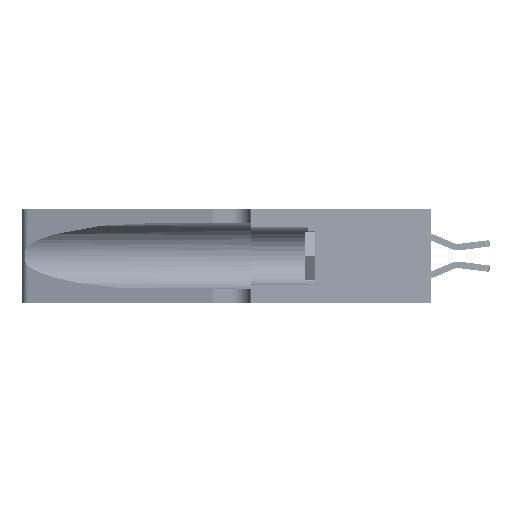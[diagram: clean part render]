
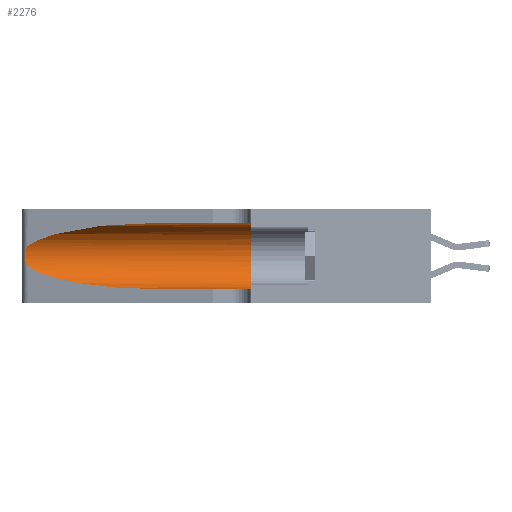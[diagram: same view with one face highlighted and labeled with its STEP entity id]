
A CAD part, left-side view. The second image highlights one B-rep face of the part: STEP entity #2276.
In plain terms, the highlighted cylindrical face has radius 3.308 mm (diameter 6.617 mm), a partial arc.
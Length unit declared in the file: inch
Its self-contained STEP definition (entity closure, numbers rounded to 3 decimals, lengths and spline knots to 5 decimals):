
#54 = B_SPLINE_CURVE_WITH_KNOTS ( 'NONE', 3,
 ( #20514, #29597, #14233, #14627, #8678, #23740, #5501, #35962, #20780, #38683, #17719, #36096, #39072, #2521 ),
 .UNSPECIFIED., .F., .F.,
 ( 4, 2, 2, 2, 2, 2, 4 ),
 ( 0., 0.00027, 0.00053, 0.00107, 0.0016, 0.00187, 0.00214 ),
 .UNSPECIFIED. ) ;
#2276 = ADVANCED_FACE ( 'NONE', ( #38828 ), #4067, .F. ) ;
#2521 = CARTESIAN_POINT ( 'NONE',  ( 0.25487, 1.22718, 0.14631 ) ) ;
#2707 = CARTESIAN_POINT ( 'NONE',  ( 0.2373, 1.15595, 0.28018 ) ) ;
#2914 = CARTESIAN_POINT ( 'NONE',  ( 0.25487, 1.22718, 0.22369 ) ) ;
#3905 = EDGE_CURVE ( 'NONE', #10264, #30009, #9099, .T. ) ;
#4067 = CYLINDRICAL_SURFACE ( 'NONE', #34800, 0.13025 ) ;
#4420 = CARTESIAN_POINT ( 'NONE',  ( 0.1305, 0.72297, 0.05475 ) ) ;
#5406 = VERTEX_POINT ( 'NONE', #33370 ) ;
#5501 = CARTESIAN_POINT ( 'NONE',  ( 0.26075, 1.23896, 0.19203 ) ) ;
#5690 = EDGE_CURVE ( 'NONE', #30009, #9125, #54, .T. ) ;
#7282 = LINE ( 'NONE', #33819, #27696 ) ;
#7378 = AXIS2_PLACEMENT_3D ( 'NONE', #16322, #13257, #22355 ) ;
#7636 = CARTESIAN_POINT ( 'NONE',  ( 0.1305, 1.61858, 0.185 ) ) ;
#8006 = CARTESIAN_POINT ( 'NONE',  ( 0.18966, 0.96281, 0.05475 ) ) ;
#8263 = VERTEX_POINT ( 'NONE', #22539 ) ;
#8368 = VECTOR ( 'NONE', #34060, 39.37008 ) ;
#8678 = CARTESIAN_POINT ( 'NONE',  ( 0.25854, 1.2359, 0.20912 ) ) ;
#9099 =( BOUNDED_CURVE ( )  B_SPLINE_CURVE ( 3, ( #21336, #33081, #2707, #14925 ),
 .UNSPECIFIED., .F., .F. ) 
 B_SPLINE_CURVE_WITH_KNOTS ( ( 4, 4 ),
 ( 1.5708, 2.84003 ),
 .UNSPECIFIED. ) 
 CURVE ( )  GEOMETRIC_REPRESENTATION_ITEM ( )  RATIONAL_B_SPLINE_CURVE ( ( 1., 0.87, 0.87, 1. ) ) 
 REPRESENTATION_ITEM ( '' )  );
#9125 = VERTEX_POINT ( 'NONE', #16091 ) ;
#9540 = CIRCLE ( 'NONE', #7378, 0.13025 ) ;
#10264 = VERTEX_POINT ( 'NONE', #32098 ) ;
#10429 = CARTESIAN_POINT ( 'NONE',  ( 0.1305, 0.35, 0.05475 ) ) ;
#13257 = DIRECTION ( 'NONE',  ( 0., 1., 0. ) ) ;
#13817 = CARTESIAN_POINT ( 'NONE',  ( 0.25487, 1.22718, 0.14631 ) ) ;
#13848 = ORIENTED_EDGE ( 'NONE', *, *, #3905, .T. ) ;
#14233 = CARTESIAN_POINT ( 'NONE',  ( 0.25639, 1.23184, 0.21858 ) ) ;
#14627 = CARTESIAN_POINT ( 'NONE',  ( 0.25787, 1.23484, 0.2124 ) ) ;
#14925 = CARTESIAN_POINT ( 'NONE',  ( 0.25487, 1.22718, 0.22369 ) ) ;
#15424 =( BOUNDED_CURVE ( )  B_SPLINE_CURVE ( 3, ( #13817, #23204, #8006, #4420 ),
 .UNSPECIFIED., .F., .F. ) 
 B_SPLINE_CURVE_WITH_KNOTS ( ( 4, 4 ),
 ( 3.44316, 4.71239 ),
 .UNSPECIFIED. ) 
 CURVE ( )  GEOMETRIC_REPRESENTATION_ITEM ( )  RATIONAL_B_SPLINE_CURVE ( ( 1., 0.87, 0.87, 1. ) ) 
 REPRESENTATION_ITEM ( '' )  );
#15707 = DIRECTION ( 'NONE',  ( 0., -1., 0. ) ) ;
#16091 = CARTESIAN_POINT ( 'NONE',  ( 0.25487, 1.22718, 0.14631 ) ) ;
#16322 = CARTESIAN_POINT ( 'NONE',  ( 0.1305, 0.35, 0.185 ) ) ;
#17719 = CARTESIAN_POINT ( 'NONE',  ( 0.25789, 1.23486, 0.15765 ) ) ;
#19360 = ORIENTED_EDGE ( 'NONE', *, *, #34183, .F. ) ;
#20514 = CARTESIAN_POINT ( 'NONE',  ( 0.25487, 1.22718, 0.22369 ) ) ;
#20580 = EDGE_CURVE ( 'NONE', #8263, #33187, #7282, .T. ) ;
#20780 = CARTESIAN_POINT ( 'NONE',  ( 0.26017, 1.23833, 0.17102 ) ) ;
#21336 = CARTESIAN_POINT ( 'NONE',  ( 0.1305, 0.72297, 0.31525 ) ) ;
#21684 = LINE ( 'NONE', #27854, #8368 ) ;
#22126 = ORIENTED_EDGE ( 'NONE', *, *, #29719, .T. ) ;
#22355 = DIRECTION ( 'NONE',  ( 0., 0., 1. ) ) ;
#22539 = CARTESIAN_POINT ( 'NONE',  ( 0.1305, 0.72297, 0.05475 ) ) ;
#22806 = DIRECTION ( 'NONE',  ( 0., 0., -1. ) ) ;
#23204 = CARTESIAN_POINT ( 'NONE',  ( 0.2373, 1.15595, 0.08982 ) ) ;
#23545 = ORIENTED_EDGE ( 'NONE', *, *, #5690, .T. ) ;
#23740 = CARTESIAN_POINT ( 'NONE',  ( 0.26018, 1.23835, 0.19895 ) ) ;
#27354 = EDGE_LOOP ( 'NONE', ( #13848, #23545, #22126, #30783, #37189, #19360 ) ) ;
#27696 = VECTOR ( 'NONE', #15707, 39.37008 ) ;
#27854 = CARTESIAN_POINT ( 'NONE',  ( 0.1305, 1.61858, 0.31525 ) ) ;
#29597 = CARTESIAN_POINT ( 'NONE',  ( 0.25555, 1.22994, 0.2215 ) ) ;
#29719 = EDGE_CURVE ( 'NONE', #9125, #8263, #15424, .T. ) ;
#30009 = VERTEX_POINT ( 'NONE', #2914 ) ;
#30223 = EDGE_CURVE ( 'NONE', #5406, #33187, #9540, .T. ) ;
#30783 = ORIENTED_EDGE ( 'NONE', *, *, #20580, .T. ) ;
#32098 = CARTESIAN_POINT ( 'NONE',  ( 0.1305, 0.72297, 0.31525 ) ) ;
#33081 = CARTESIAN_POINT ( 'NONE',  ( 0.18966, 0.96281, 0.31525 ) ) ;
#33187 = VERTEX_POINT ( 'NONE', #10429 ) ;
#33370 = CARTESIAN_POINT ( 'NONE',  ( 0.1305, 0.35, 0.31525 ) ) ;
#33819 = CARTESIAN_POINT ( 'NONE',  ( 0.1305, 1.61858, 0.05475 ) ) ;
#34060 = DIRECTION ( 'NONE',  ( 0., -1., 0. ) ) ;
#34183 = EDGE_CURVE ( 'NONE', #10264, #5406, #21684, .T. ) ;
#34800 = AXIS2_PLACEMENT_3D ( 'NONE', #7636, #34904, #22806 ) ;
#34904 = DIRECTION ( 'NONE',  ( 0., -1., 0. ) ) ;
#35962 = CARTESIAN_POINT ( 'NONE',  ( 0.26075, 1.23896, 0.178 ) ) ;
#36096 = CARTESIAN_POINT ( 'NONE',  ( 0.25639, 1.23186, 0.15144 ) ) ;
#37189 = ORIENTED_EDGE ( 'NONE', *, *, #30223, .F. ) ;
#38683 = CARTESIAN_POINT ( 'NONE',  ( 0.25856, 1.23593, 0.16098 ) ) ;
#38828 = FACE_OUTER_BOUND ( 'NONE', #27354, .T. ) ;
#39072 = CARTESIAN_POINT ( 'NONE',  ( 0.25555, 1.22993, 0.14849 ) ) ;
